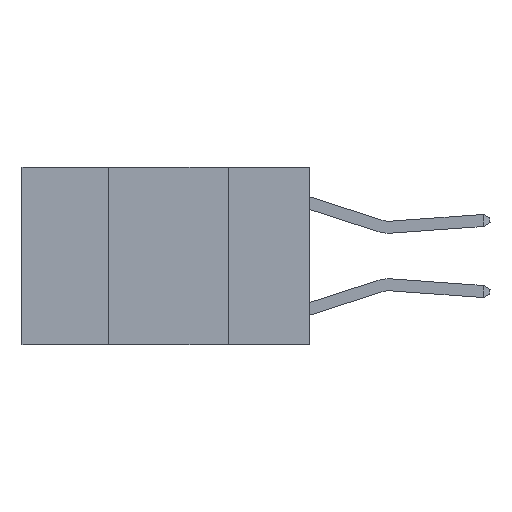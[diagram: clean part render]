
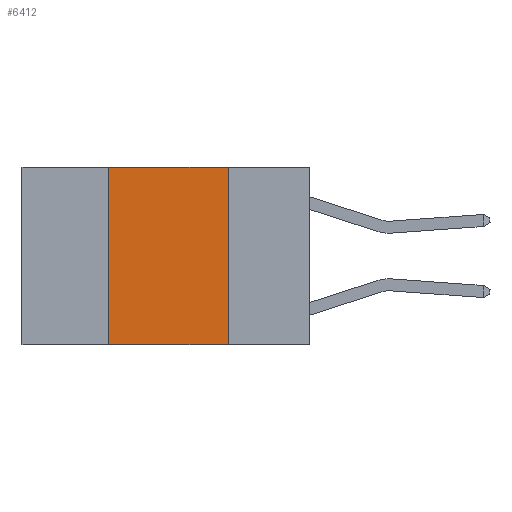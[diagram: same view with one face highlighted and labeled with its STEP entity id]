
A CAD part, left-side view. The second image highlights one B-rep face of the part: STEP entity #6412.
In plain terms, the highlighted planar face has unit normal (-1, 0, 0).
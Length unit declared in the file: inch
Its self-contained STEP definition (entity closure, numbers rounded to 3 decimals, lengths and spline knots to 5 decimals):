
#360 = CARTESIAN_POINT ( 'NONE',  ( 0., 0.17, 0. ) ) ;
#899 = CARTESIAN_POINT ( 'NONE',  ( 0., 0.42, 0. ) ) ;
#1837 = DIRECTION ( 'NONE',  ( 0., -1., 0. ) ) ;
#2607 = CARTESIAN_POINT ( 'NONE',  ( 0., 0.42, 0. ) ) ;
#3320 = EDGE_CURVE ( 'NONE', #19621, #5335, #8147, .T. ) ;
#4954 = AXIS2_PLACEMENT_3D ( 'NONE', #25029, #17040, #7350 ) ;
#4963 = DIRECTION ( 'NONE',  ( 0., 0., -1. ) ) ;
#5008 = EDGE_LOOP ( 'NONE', ( #20851, #5527, #20292, #20830 ) ) ;
#5335 = VERTEX_POINT ( 'NONE', #12779 ) ;
#5527 = ORIENTED_EDGE ( 'NONE', *, *, #20498, .F. ) ;
#6412 = ADVANCED_FACE ( 'NONE', ( #17156 ), #9284, .F. ) ;
#6482 = VERTEX_POINT ( 'NONE', #360 ) ;
#7350 = DIRECTION ( 'NONE',  ( 0., 0., -1. ) ) ;
#7788 = CARTESIAN_POINT ( 'NONE',  ( 0., 0.42, -0.37 ) ) ;
#7829 = LINE ( 'NONE', #23454, #23059 ) ;
#8147 = LINE ( 'NONE', #12289, #12694 ) ;
#8205 = DIRECTION ( 'NONE',  ( 0., -1., 0. ) ) ;
#9284 = PLANE ( 'NONE',  #4954 ) ;
#12271 = LINE ( 'NONE', #899, #21892 ) ;
#12289 = CARTESIAN_POINT ( 'NONE',  ( 0., 0.6, -0.37 ) ) ;
#12694 = VECTOR ( 'NONE', #1837, 39.37008 ) ;
#12731 = LINE ( 'NONE', #18752, #20406 ) ;
#12779 = CARTESIAN_POINT ( 'NONE',  ( 0., 0.17, -0.37 ) ) ;
#14106 = EDGE_CURVE ( 'NONE', #6482, #5335, #12731, .T. ) ;
#17040 = DIRECTION ( 'NONE',  ( 1., 0., 0. ) ) ;
#17156 = FACE_OUTER_BOUND ( 'NONE', #5008, .T. ) ;
#18183 = DIRECTION ( 'NONE',  ( 0., 0., 1. ) ) ;
#18752 = CARTESIAN_POINT ( 'NONE',  ( 0., 0.17, 0. ) ) ;
#18956 = VERTEX_POINT ( 'NONE', #2607 ) ;
#19621 = VERTEX_POINT ( 'NONE', #7788 ) ;
#20292 = ORIENTED_EDGE ( 'NONE', *, *, #24130, .F. ) ;
#20406 = VECTOR ( 'NONE', #4963, 39.37008 ) ;
#20498 = EDGE_CURVE ( 'NONE', #18956, #6482, #7829, .T. ) ;
#20830 = ORIENTED_EDGE ( 'NONE', *, *, #3320, .T. ) ;
#20851 = ORIENTED_EDGE ( 'NONE', *, *, #14106, .F. ) ;
#21892 = VECTOR ( 'NONE', #18183, 39.37008 ) ;
#23059 = VECTOR ( 'NONE', #8205, 39.37008 ) ;
#23454 = CARTESIAN_POINT ( 'NONE',  ( 0., 0.6, 0. ) ) ;
#24130 = EDGE_CURVE ( 'NONE', #19621, #18956, #12271, .T. ) ;
#25029 = CARTESIAN_POINT ( 'NONE',  ( 0., 0.6, 0. ) ) ;
